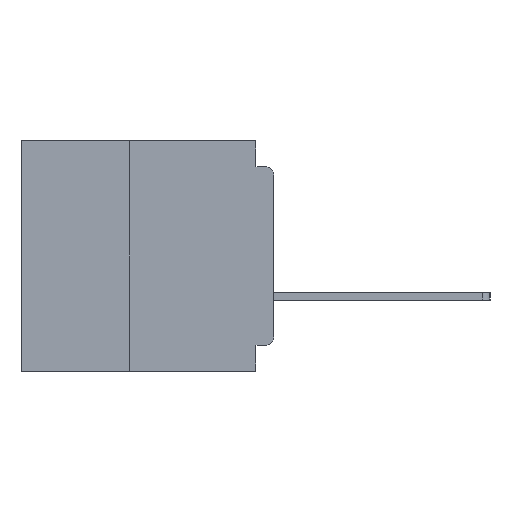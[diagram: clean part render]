
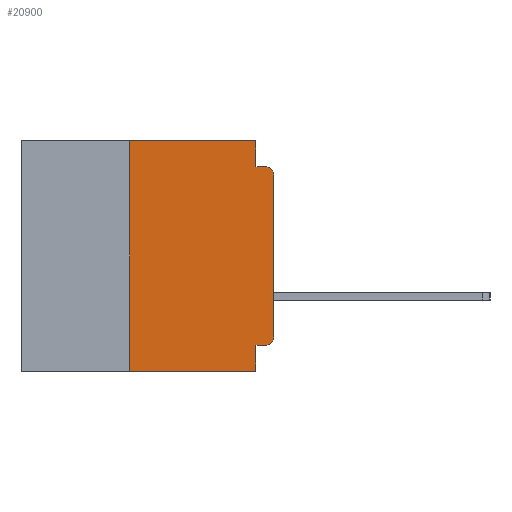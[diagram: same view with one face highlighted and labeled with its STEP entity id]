
A CAD part, left-side view. The second image highlights one B-rep face of the part: STEP entity #20900.
In plain terms, the highlighted planar face has unit normal (-1, 0, 0).
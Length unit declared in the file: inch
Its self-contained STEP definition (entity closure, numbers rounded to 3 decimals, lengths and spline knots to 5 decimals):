
#21 = VECTOR ( 'NONE', #10092, 39.37008 ) ;
#209 = CARTESIAN_POINT ( 'NONE',  ( 0., 0.437, 0. ) ) ;
#352 = DIRECTION ( 'NONE',  ( 1., 0., 0. ) ) ;
#401 = VECTOR ( 'NONE', #5173, 39.37008 ) ;
#478 = CIRCLE ( 'NONE', #28797, 0.015 ) ;
#1154 = EDGE_CURVE ( 'NONE', #35877, #3724, #25680, .T. ) ;
#1606 = CARTESIAN_POINT ( 'NONE',  ( 0., 0.031, -0.355 ) ) ;
#1844 = EDGE_CURVE ( 'NONE', #37835, #15335, #478, .T. ) ;
#2110 = DIRECTION ( 'NONE',  ( 0., -1., 0. ) ) ;
#3177 = EDGE_CURVE ( 'NONE', #40355, #37835, #30917, .T. ) ;
#3333 = VERTEX_POINT ( 'NONE', #40053 ) ;
#3502 = FACE_OUTER_BOUND ( 'NONE', #18335, .T. ) ;
#3575 = CARTESIAN_POINT ( 'NONE',  ( 0., 0.015, -0.06 ) ) ;
#3724 = VERTEX_POINT ( 'NONE', #8721 ) ;
#3758 = CARTESIAN_POINT ( 'NONE',  ( 0., 0.031, 0. ) ) ;
#4217 = LINE ( 'NONE', #32891, #11804 ) ;
#4530 = EDGE_CURVE ( 'NONE', #13282, #32935, #4217, .T. ) ;
#4605 = DIRECTION ( 'NONE',  ( -1., 0., 0. ) ) ;
#5173 = DIRECTION ( 'NONE',  ( 0., 0., -1. ) ) ;
#5720 = CARTESIAN_POINT ( 'NONE',  ( 0., 0.25, -0.4 ) ) ;
#6051 = VECTOR ( 'NONE', #16032, 39.37008 ) ;
#6095 = EDGE_CURVE ( 'NONE', #14440, #35877, #23201, .T. ) ;
#7443 = ORIENTED_EDGE ( 'NONE', *, *, #3177, .T. ) ;
#8083 = CIRCLE ( 'NONE', #25865, 0.015 ) ;
#8721 = CARTESIAN_POINT ( 'NONE',  ( 0., 0.031, -0.4 ) ) ;
#8942 = LINE ( 'NONE', #24476, #401 ) ;
#9057 = VECTOR ( 'NONE', #31363, 39.37008 ) ;
#9560 = CARTESIAN_POINT ( 'NONE',  ( 0., 0., -0.355 ) ) ;
#9923 = PLANE ( 'NONE',  #21840 ) ;
#10092 = DIRECTION ( 'NONE',  ( 0., 0., -1. ) ) ;
#10392 = CARTESIAN_POINT ( 'NONE',  ( 0., 0.031, -0.4 ) ) ;
#11367 = ORIENTED_EDGE ( 'NONE', *, *, #4530, .F. ) ;
#11804 = VECTOR ( 'NONE', #32800, 39.37008 ) ;
#11907 = VECTOR ( 'NONE', #2110, 39.37008 ) ;
#12403 = CARTESIAN_POINT ( 'NONE',  ( 0., 0.015, -0.045 ) ) ;
#12483 = ORIENTED_EDGE ( 'NONE', *, *, #30918, .F. ) ;
#12779 = CARTESIAN_POINT ( 'NONE',  ( 0., 0.031, -0.045 ) ) ;
#12890 = LINE ( 'NONE', #40459, #11907 ) ;
#13282 = VERTEX_POINT ( 'NONE', #34690 ) ;
#13621 = DIRECTION ( 'NONE',  ( 0., -1., 0. ) ) ;
#13679 = LINE ( 'NONE', #32716, #40169 ) ;
#14291 = EDGE_CURVE ( 'NONE', #3333, #3724, #13679, .T. ) ;
#14325 = ORIENTED_EDGE ( 'NONE', *, *, #1154, .F. ) ;
#14440 = VERTEX_POINT ( 'NONE', #17369 ) ;
#15217 = ORIENTED_EDGE ( 'NONE', *, *, #27668, .F. ) ;
#15335 = VERTEX_POINT ( 'NONE', #12403 ) ;
#15444 = ORIENTED_EDGE ( 'NONE', *, *, #30541, .T. ) ;
#16032 = DIRECTION ( 'NONE',  ( 0., 1., 0. ) ) ;
#17145 = ORIENTED_EDGE ( 'NONE', *, *, #1844, .T. ) ;
#17369 = CARTESIAN_POINT ( 'NONE',  ( 0., 0.015, -0.355 ) ) ;
#18335 = EDGE_LOOP ( 'NONE', ( #7443, #17145, #15217, #31236, #11367, #12483, #23504, #14325, #31767, #15444 ) ) ;
#20900 = ADVANCED_FACE ( 'NONE', ( #3502 ), #9923, .F. ) ;
#21840 = AXIS2_PLACEMENT_3D ( 'NONE', #209, #352, #22837 ) ;
#21956 = VERTEX_POINT ( 'NONE', #12779 ) ;
#22470 = VECTOR ( 'NONE', #29134, 39.37008 ) ;
#22837 = DIRECTION ( 'NONE',  ( 0., 0., -1. ) ) ;
#23201 = LINE ( 'NONE', #9560, #6051 ) ;
#23504 = ORIENTED_EDGE ( 'NONE', *, *, #14291, .T. ) ;
#23888 = CARTESIAN_POINT ( 'NONE',  ( 0., 0.015, -0.34 ) ) ;
#24476 = CARTESIAN_POINT ( 'NONE',  ( 0., 0.031, 0. ) ) ;
#25680 = LINE ( 'NONE', #10392, #21 ) ;
#25865 = AXIS2_PLACEMENT_3D ( 'NONE', #23888, #4605, #27096 ) ;
#27096 = DIRECTION ( 'NONE',  ( 0., 0., -1. ) ) ;
#27668 = EDGE_CURVE ( 'NONE', #21956, #15335, #12890, .T. ) ;
#28797 = AXIS2_PLACEMENT_3D ( 'NONE', #3575, #40960, #39245 ) ;
#29134 = DIRECTION ( 'NONE',  ( 0., 0., 1. ) ) ;
#30541 = EDGE_CURVE ( 'NONE', #14440, #40355, #8083, .T. ) ;
#30735 = CARTESIAN_POINT ( 'NONE',  ( 0., 0., 0. ) ) ;
#30917 = LINE ( 'NONE', #30735, #22470 ) ;
#30918 = EDGE_CURVE ( 'NONE', #3333, #13282, #34576, .T. ) ;
#31236 = ORIENTED_EDGE ( 'NONE', *, *, #37521, .F. ) ;
#31363 = DIRECTION ( 'NONE',  ( 0., 0., 1. ) ) ;
#31767 = ORIENTED_EDGE ( 'NONE', *, *, #6095, .F. ) ;
#32716 = CARTESIAN_POINT ( 'NONE',  ( 0., 0.437, -0.4 ) ) ;
#32800 = DIRECTION ( 'NONE',  ( 0., -1., 0. ) ) ;
#32891 = CARTESIAN_POINT ( 'NONE',  ( 0., 0.437, 0. ) ) ;
#32935 = VERTEX_POINT ( 'NONE', #3758 ) ;
#34576 = LINE ( 'NONE', #5720, #9057 ) ;
#34690 = CARTESIAN_POINT ( 'NONE',  ( 0., 0.25, 0. ) ) ;
#35877 = VERTEX_POINT ( 'NONE', #1606 ) ;
#37521 = EDGE_CURVE ( 'NONE', #32935, #21956, #8942, .T. ) ;
#37835 = VERTEX_POINT ( 'NONE', #39033 ) ;
#39033 = CARTESIAN_POINT ( 'NONE',  ( 0., 0., -0.06 ) ) ;
#39245 = DIRECTION ( 'NONE',  ( 0., 0., -1. ) ) ;
#40053 = CARTESIAN_POINT ( 'NONE',  ( 0., 0.25, -0.4 ) ) ;
#40169 = VECTOR ( 'NONE', #13621, 39.37008 ) ;
#40355 = VERTEX_POINT ( 'NONE', #41336 ) ;
#40459 = CARTESIAN_POINT ( 'NONE',  ( 0., 0., -0.045 ) ) ;
#40960 = DIRECTION ( 'NONE',  ( -1., 0., 0. ) ) ;
#41336 = CARTESIAN_POINT ( 'NONE',  ( 0., 0., -0.34 ) ) ;
